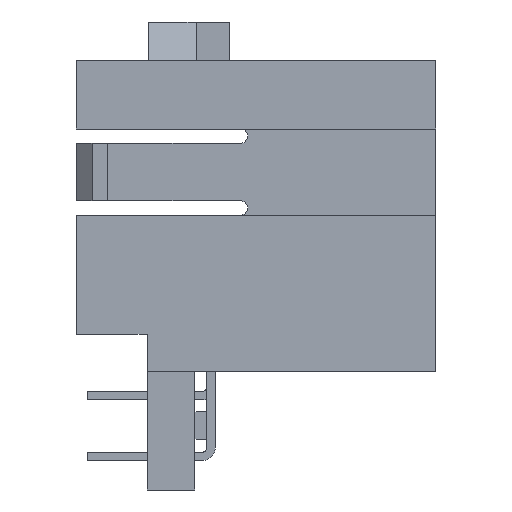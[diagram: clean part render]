
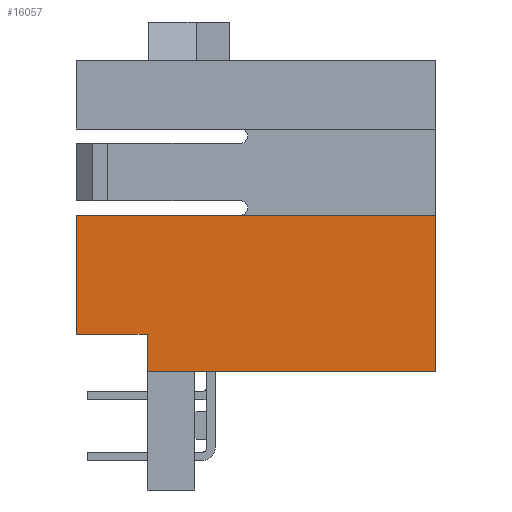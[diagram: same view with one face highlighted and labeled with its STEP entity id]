
A CAD part, left-side view. The second image highlights one B-rep face of the part: STEP entity #16057.
In plain terms, the highlighted planar face has unit normal (-1, 0, 0).
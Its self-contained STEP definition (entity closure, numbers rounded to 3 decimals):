
#371 = LINE ( 'NONE', #1966, #4168 ) ;
#390 = ORIENTED_EDGE ( 'NONE', *, *, #1856, .T. ) ;
#426 = VECTOR ( 'NONE', #12428, 1000. ) ;
#1083 = CARTESIAN_POINT ( 'NONE',  ( -7.6, 15., 0.03 ) ) ;
#1147 = CARTESIAN_POINT ( 'NONE',  ( -7.6, 0., -6.5 ) ) ;
#1248 = LINE ( 'NONE', #17562, #3051 ) ;
#1318 = LINE ( 'NONE', #13563, #4221 ) ;
#1546 = DIRECTION ( 'NONE',  ( 0., 0., 1. ) ) ;
#1856 = EDGE_CURVE ( 'NONE', #1981, #8657, #1318, .T. ) ;
#1966 = CARTESIAN_POINT ( 'NONE',  ( -7.6, 7.5, 0.03 ) ) ;
#1972 = EDGE_CURVE ( 'NONE', #18657, #1981, #2450, .T. ) ;
#1981 = VERTEX_POINT ( 'NONE', #1147 ) ;
#2450 = LINE ( 'NONE', #12487, #426 ) ;
#3051 = VECTOR ( 'NONE', #8899, 1000. ) ;
#3110 = ORIENTED_EDGE ( 'NONE', *, *, #3189, .T. ) ;
#3189 = EDGE_CURVE ( 'NONE', #8657, #12514, #371, .T. ) ;
#3233 = DIRECTION ( 'NONE',  ( 0., 0., -1. ) ) ;
#3442 = EDGE_CURVE ( 'NONE', #4113, #11740, #4947, .T. ) ;
#3642 = VECTOR ( 'NONE', #4131, 1000. ) ;
#4113 = VERTEX_POINT ( 'NONE', #10282 ) ;
#4131 = DIRECTION ( 'NONE',  ( 0., 1., 0. ) ) ;
#4168 = VECTOR ( 'NONE', #6493, 1000. ) ;
#4221 = VECTOR ( 'NONE', #10862, 1000. ) ;
#4295 = CARTESIAN_POINT ( 'NONE',  ( -7.6, -0.3, -6.76 ) ) ;
#4947 = LINE ( 'NONE', #6843, #3642 ) ;
#5037 = ORIENTED_EDGE ( 'NONE', *, *, #14043, .F. ) ;
#5583 = CARTESIAN_POINT ( 'NONE',  ( -7.6, 0., 0.03 ) ) ;
#5616 = AXIS2_PLACEMENT_3D ( 'NONE', #4295, #13066, #1546 ) ;
#6493 = DIRECTION ( 'NONE',  ( 0., 1., 0. ) ) ;
#6843 = CARTESIAN_POINT ( 'NONE',  ( -7.6, 13.525, -4.95 ) ) ;
#7543 = ORIENTED_EDGE ( 'NONE', *, *, #10080, .T. ) ;
#7752 = ORIENTED_EDGE ( 'NONE', *, *, #1972, .T. ) ;
#8116 = CARTESIAN_POINT ( 'NONE',  ( -7.6, 12.05, -6.5 ) ) ;
#8657 = VERTEX_POINT ( 'NONE', #5583 ) ;
#8701 = CARTESIAN_POINT ( 'NONE',  ( -7.6, 12.05, 0. ) ) ;
#8899 = DIRECTION ( 'NONE',  ( 0., 0., 1. ) ) ;
#10080 = EDGE_CURVE ( 'NONE', #4113, #18657, #12488, .T. ) ;
#10242 = EDGE_LOOP ( 'NONE', ( #7752, #390, #3110, #5037, #16142, #7543 ) ) ;
#10282 = CARTESIAN_POINT ( 'NONE',  ( -7.6, 12.05, -4.95 ) ) ;
#10862 = DIRECTION ( 'NONE',  ( 0., 0., 1. ) ) ;
#11740 = VERTEX_POINT ( 'NONE', #13744 ) ;
#12428 = DIRECTION ( 'NONE',  ( 0., -1., 0. ) ) ;
#12487 = CARTESIAN_POINT ( 'NONE',  ( -7.6, 7.5, -6.5 ) ) ;
#12488 = LINE ( 'NONE', #8701, #15649 ) ;
#12514 = VERTEX_POINT ( 'NONE', #1083 ) ;
#12936 = PLANE ( 'NONE',  #5616 ) ;
#13066 = DIRECTION ( 'NONE',  ( -1., 0., 0. ) ) ;
#13563 = CARTESIAN_POINT ( 'NONE',  ( -7.6, 0., 0. ) ) ;
#13744 = CARTESIAN_POINT ( 'NONE',  ( -7.6, 15., -4.95 ) ) ;
#14043 = EDGE_CURVE ( 'NONE', #11740, #12514, #1248, .T. ) ;
#14706 = FACE_OUTER_BOUND ( 'NONE', #10242, .T. ) ;
#15649 = VECTOR ( 'NONE', #3233, 1000. ) ;
#16057 = ADVANCED_FACE ( 'NONE', ( #14706 ), #12936, .T. ) ;
#16142 = ORIENTED_EDGE ( 'NONE', *, *, #3442, .F. ) ;
#17562 = CARTESIAN_POINT ( 'NONE',  ( -7.6, 15., 0.775 ) ) ;
#18657 = VERTEX_POINT ( 'NONE', #8116 ) ;
